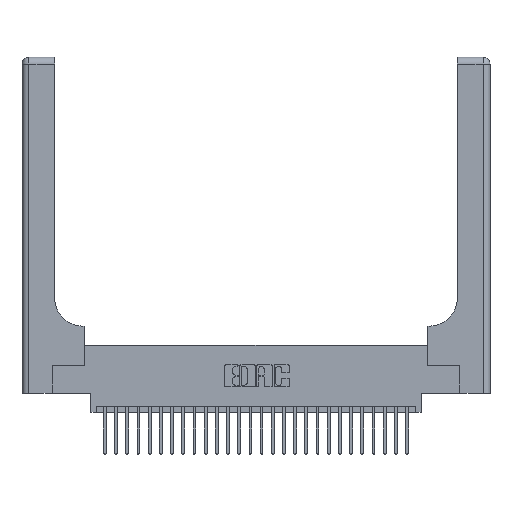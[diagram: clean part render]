
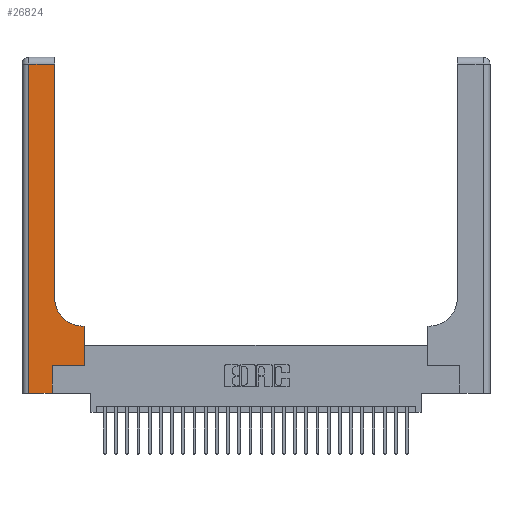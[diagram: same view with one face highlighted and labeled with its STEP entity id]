
A CAD part, top view. The second image highlights one B-rep face of the part: STEP entity #26824.
In plain terms, the highlighted planar face has unit normal (0, 0, 1).
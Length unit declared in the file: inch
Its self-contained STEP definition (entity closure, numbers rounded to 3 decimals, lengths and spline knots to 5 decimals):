
#647 = CARTESIAN_POINT ( 'NONE',  ( 0.5415, 0.85, 0.37 ) ) ;
#1895 = VECTOR ( 'NONE', #18859, 39.37008 ) ;
#2033 = VECTOR ( 'NONE', #13167, 39.37008 ) ;
#3098 = CARTESIAN_POINT ( 'NONE',  ( 0.5585, 0.25, 0.37 ) ) ;
#3119 = LINE ( 'NONE', #13196, #17944 ) ;
#3652 = EDGE_CURVE ( 'NONE', #6205, #22695, #11950, .T. ) ;
#3738 = ORIENTED_EDGE ( 'NONE', *, *, #6054, .T. ) ;
#4345 = VECTOR ( 'NONE', #28462, 39.37008 ) ;
#4661 = PLANE ( 'NONE',  #11536 ) ;
#4924 = EDGE_CURVE ( 'NONE', #21349, #11862, #20032, .T. ) ;
#5052 = CARTESIAN_POINT ( 'NONE',  ( 0.269, 0., 0.37 ) ) ;
#5086 = DIRECTION ( 'NONE',  ( 1., 0., 0. ) ) ;
#5427 = VERTEX_POINT ( 'NONE', #16427 ) ;
#5482 = CARTESIAN_POINT ( 'NONE',  ( 0.06, 0., 0.37 ) ) ;
#6054 = EDGE_CURVE ( 'NONE', #19951, #5427, #6909, .T. ) ;
#6205 = VERTEX_POINT ( 'NONE', #25922 ) ;
#6581 = DIRECTION ( 'NONE',  ( -1., 0., 0. ) ) ;
#6909 = LINE ( 'NONE', #16632, #15423 ) ;
#7795 = ORIENTED_EDGE ( 'NONE', *, *, #20056, .T. ) ;
#7807 = EDGE_CURVE ( 'NONE', #5427, #8303, #15653, .T. ) ;
#7825 = CARTESIAN_POINT ( 'NONE',  ( 0.5585, 0.25, 0.37 ) ) ;
#7881 = ORIENTED_EDGE ( 'NONE', *, *, #11576, .T. ) ;
#8245 = ORIENTED_EDGE ( 'NONE', *, *, #3652, .T. ) ;
#8303 = VERTEX_POINT ( 'NONE', #7825 ) ;
#8377 = LINE ( 'NONE', #23694, #17202 ) ;
#8733 = DIRECTION ( 'NONE',  ( 0., -1., 0. ) ) ;
#8831 = FACE_OUTER_BOUND ( 'NONE', #25993, .T. ) ;
#8886 = CIRCLE ( 'NONE', #27646, 0.25 ) ;
#8900 = CARTESIAN_POINT ( 'NONE',  ( 0., 3., 0.37 ) ) ;
#9336 = CARTESIAN_POINT ( 'NONE',  ( 0.06, 2.94, 0.37 ) ) ;
#9625 = CARTESIAN_POINT ( 'NONE',  ( 0.5585, 0.6, 0.37 ) ) ;
#11105 = ORIENTED_EDGE ( 'NONE', *, *, #17106, .T. ) ;
#11536 = AXIS2_PLACEMENT_3D ( 'NONE', #8900, #15900, #6581 ) ;
#11576 = EDGE_CURVE ( 'NONE', #14895, #19951, #26798, .T. ) ;
#11862 = VERTEX_POINT ( 'NONE', #12193 ) ;
#11950 = LINE ( 'NONE', #28424, #20423 ) ;
#12193 = CARTESIAN_POINT ( 'NONE',  ( 0.5415, 0.6, 0.37 ) ) ;
#12696 = CARTESIAN_POINT ( 'NONE',  ( 0.269, 0.25, 0.37 ) ) ;
#12870 = EDGE_CURVE ( 'NONE', #15968, #6205, #8377, .T. ) ;
#12879 = CARTESIAN_POINT ( 'NONE',  ( 0.2915, 0.6, 0.37 ) ) ;
#12965 = DIRECTION ( 'NONE',  ( -1., 0., 0. ) ) ;
#13167 = DIRECTION ( 'NONE',  ( -1., 0., 0. ) ) ;
#13196 = CARTESIAN_POINT ( 'NONE',  ( 0.06, 3., 0.37 ) ) ;
#14895 = VERTEX_POINT ( 'NONE', #5482 ) ;
#15423 = VECTOR ( 'NONE', #16547, 39.37008 ) ;
#15653 = LINE ( 'NONE', #12696, #4345 ) ;
#15900 = DIRECTION ( 'NONE',  ( 0., 0., -1. ) ) ;
#15968 = VERTEX_POINT ( 'NONE', #16565 ) ;
#16427 = CARTESIAN_POINT ( 'NONE',  ( 0.269, 0.25, 0.37 ) ) ;
#16547 = DIRECTION ( 'NONE',  ( 0., 1., 0. ) ) ;
#16565 = CARTESIAN_POINT ( 'NONE',  ( 0.2915, 0.85, 0.37 ) ) ;
#16632 = CARTESIAN_POINT ( 'NONE',  ( 0.269, 0., 0.37 ) ) ;
#16651 = ORIENTED_EDGE ( 'NONE', *, *, #4924, .T. ) ;
#16754 = CARTESIAN_POINT ( 'NONE',  ( 0., 0., 0.37 ) ) ;
#17106 = EDGE_CURVE ( 'NONE', #22695, #14895, #3119, .T. ) ;
#17202 = VECTOR ( 'NONE', #18962, 39.37008 ) ;
#17944 = VECTOR ( 'NONE', #8733, 39.37008 ) ;
#18680 = DIRECTION ( 'NONE',  ( 0., 0., -1. ) ) ;
#18859 = DIRECTION ( 'NONE',  ( 0., 1., 0. ) ) ;
#18962 = DIRECTION ( 'NONE',  ( 0., 1., 0. ) ) ;
#19951 = VERTEX_POINT ( 'NONE', #5052 ) ;
#20032 = LINE ( 'NONE', #12879, #2033 ) ;
#20056 = EDGE_CURVE ( 'NONE', #8303, #21349, #26567, .T. ) ;
#20423 = VECTOR ( 'NONE', #12965, 39.37008 ) ;
#21247 = EDGE_CURVE ( 'NONE', #11862, #15968, #8886, .T. ) ;
#21349 = VERTEX_POINT ( 'NONE', #9625 ) ;
#22695 = VERTEX_POINT ( 'NONE', #9336 ) ;
#23216 = ORIENTED_EDGE ( 'NONE', *, *, #21247, .T. ) ;
#23694 = CARTESIAN_POINT ( 'NONE',  ( 0.2915, 3., 0.37 ) ) ;
#24259 = ORIENTED_EDGE ( 'NONE', *, *, #12870, .T. ) ;
#25367 = VECTOR ( 'NONE', #26207, 39.37008 ) ;
#25922 = CARTESIAN_POINT ( 'NONE',  ( 0.2915, 2.94, 0.37 ) ) ;
#25993 = EDGE_LOOP ( 'NONE', ( #24259, #8245, #11105, #7881, #3738, #27451, #7795, #16651, #23216 ) ) ;
#26207 = DIRECTION ( 'NONE',  ( 1., 0., 0. ) ) ;
#26567 = LINE ( 'NONE', #3098, #1895 ) ;
#26798 = LINE ( 'NONE', #16754, #25367 ) ;
#26824 = ADVANCED_FACE ( 'NONE', ( #8831 ), #4661, .F. ) ;
#27451 = ORIENTED_EDGE ( 'NONE', *, *, #7807, .T. ) ;
#27646 = AXIS2_PLACEMENT_3D ( 'NONE', #647, #18680, #5086 ) ;
#28424 = CARTESIAN_POINT ( 'NONE',  ( 0., 2.94, 0.37 ) ) ;
#28462 = DIRECTION ( 'NONE',  ( 1., 0., 0. ) ) ;
